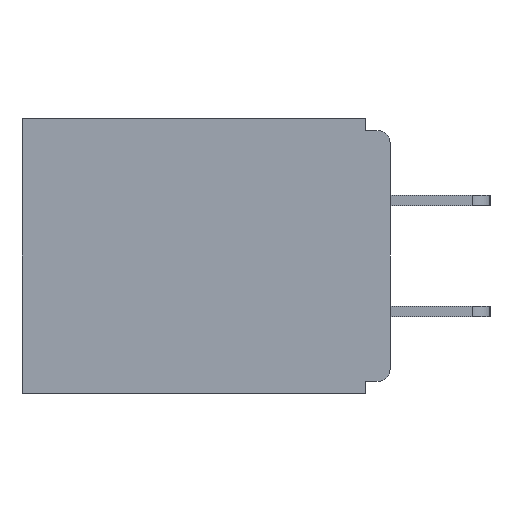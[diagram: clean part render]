
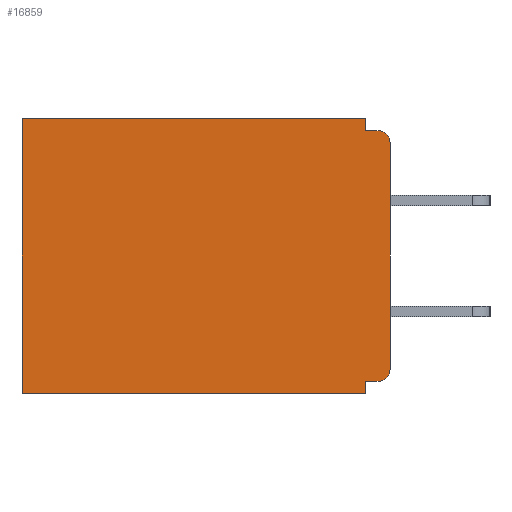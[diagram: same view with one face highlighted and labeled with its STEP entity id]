
A CAD part, left-side view. The second image highlights one B-rep face of the part: STEP entity #16859.
In plain terms, the highlighted planar face has unit normal (-1, 0, 0).
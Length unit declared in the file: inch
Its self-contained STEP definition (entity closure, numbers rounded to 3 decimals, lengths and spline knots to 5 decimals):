
#221 = EDGE_CURVE ( 'NONE', #4539, #14338, #4258, .T. ) ;
#239 = DIRECTION ( 'NONE',  ( 0., 0., -1. ) ) ;
#293 = DIRECTION ( 'NONE',  ( -1., 0., 0. ) ) ;
#510 = ORIENTED_EDGE ( 'NONE', *, *, #3918, .T. ) ;
#645 = VECTOR ( 'NONE', #3344, 39.37008 ) ;
#676 = PLANE ( 'NONE',  #13515 ) ;
#951 = ORIENTED_EDGE ( 'NONE', *, *, #10833, .F. ) ;
#1145 = ORIENTED_EDGE ( 'NONE', *, *, #6281, .T. ) ;
#1488 = CARTESIAN_POINT ( 'NONE',  ( 0.298, 0.015, -0.313 ) ) ;
#2390 = VERTEX_POINT ( 'NONE', #12334 ) ;
#2762 = EDGE_LOOP ( 'NONE', ( #510, #6011, #5870, #3075, #7403, #951, #15896, #7217, #1145, #3067 ) ) ;
#2791 = CIRCLE ( 'NONE', #11341, 0.015 ) ;
#2905 = EDGE_CURVE ( 'NONE', #3088, #14174, #4591, .T. ) ;
#3053 = AXIS2_PLACEMENT_3D ( 'NONE', #12377, #16172, #12255 ) ;
#3055 = EDGE_CURVE ( 'NONE', #2390, #16851, #3716, .T. ) ;
#3067 = ORIENTED_EDGE ( 'NONE', *, *, #2905, .F. ) ;
#3075 = ORIENTED_EDGE ( 'NONE', *, *, #9338, .T. ) ;
#3088 = VERTEX_POINT ( 'NONE', #14588 ) ;
#3344 = DIRECTION ( 'NONE',  ( 0., 1., 0. ) ) ;
#3475 = EDGE_CURVE ( 'NONE', #16851, #15355, #7860, .T. ) ;
#3716 = LINE ( 'NONE', #17116, #13738 ) ;
#3918 = EDGE_CURVE ( 'NONE', #3088, #15355, #13923, .T. ) ;
#3971 = LINE ( 'NONE', #9865, #645 ) ;
#3990 = LINE ( 'NONE', #4992, #15220 ) ;
#4104 = CARTESIAN_POINT ( 'NONE',  ( 0.298, 0.015, -0.328 ) ) ;
#4258 = LINE ( 'NONE', #12077, #7594 ) ;
#4539 = VERTEX_POINT ( 'NONE', #4104 ) ;
#4559 = LINE ( 'NONE', #13170, #6616 ) ;
#4591 = LINE ( 'NONE', #14930, #13950 ) ;
#4704 = DIRECTION ( 'NONE',  ( 0., 0., -1. ) ) ;
#4992 = CARTESIAN_POINT ( 'NONE',  ( 0.298, 0.031, -0.343 ) ) ;
#5870 = ORIENTED_EDGE ( 'NONE', *, *, #3055, .F. ) ;
#5991 = CARTESIAN_POINT ( 'NONE',  ( 0.298, 0., 0. ) ) ;
#6011 = ORIENTED_EDGE ( 'NONE', *, *, #3475, .F. ) ;
#6237 = DIRECTION ( 'NONE',  ( 0., 0., -1. ) ) ;
#6281 = EDGE_CURVE ( 'NONE', #4539, #14174, #2791, .T. ) ;
#6289 = VERTEX_POINT ( 'NONE', #13451 ) ;
#6616 = VECTOR ( 'NONE', #7856, 39.37008 ) ;
#6645 = CARTESIAN_POINT ( 'NONE',  ( 0.298, 0.46, -0.343 ) ) ;
#7136 = LINE ( 'NONE', #9548, #13598 ) ;
#7217 = ORIENTED_EDGE ( 'NONE', *, *, #221, .F. ) ;
#7403 = ORIENTED_EDGE ( 'NONE', *, *, #17065, .T. ) ;
#7594 = VECTOR ( 'NONE', #16400, 39.37008 ) ;
#7681 = CARTESIAN_POINT ( 'NONE',  ( 0.298, 0.015, -0.015 ) ) ;
#7856 = DIRECTION ( 'NONE',  ( 0., 0., -1. ) ) ;
#7860 = LINE ( 'NONE', #15106, #12038 ) ;
#8311 = DIRECTION ( 'NONE',  ( 0., 0., -1. ) ) ;
#8358 = DIRECTION ( 'NONE',  ( 0., -1., 0. ) ) ;
#8578 = CARTESIAN_POINT ( 'NONE',  ( 0.298, 0.031, -0.015 ) ) ;
#9195 = VERTEX_POINT ( 'NONE', #10672 ) ;
#9338 = EDGE_CURVE ( 'NONE', #2390, #9195, #7136, .T. ) ;
#9548 = CARTESIAN_POINT ( 'NONE',  ( 0.298, 0., 0. ) ) ;
#9865 = CARTESIAN_POINT ( 'NONE',  ( 0.298, 0., -0.343 ) ) ;
#10512 = EDGE_CURVE ( 'NONE', #14338, #6289, #3990, .T. ) ;
#10605 = VERTEX_POINT ( 'NONE', #6645 ) ;
#10672 = CARTESIAN_POINT ( 'NONE',  ( 0.298, 0.46, 0. ) ) ;
#10833 = EDGE_CURVE ( 'NONE', #6289, #10605, #3971, .T. ) ;
#11341 = AXIS2_PLACEMENT_3D ( 'NONE', #1488, #293, #239 ) ;
#12038 = VECTOR ( 'NONE', #8358, 39.37008 ) ;
#12077 = CARTESIAN_POINT ( 'NONE',  ( 0.298, 0., -0.328 ) ) ;
#12170 = CARTESIAN_POINT ( 'NONE',  ( 0.298, 0.031, -0.328 ) ) ;
#12255 = DIRECTION ( 'NONE',  ( 0., 0., -1. ) ) ;
#12334 = CARTESIAN_POINT ( 'NONE',  ( 0.298, 0.031, 0. ) ) ;
#12377 = CARTESIAN_POINT ( 'NONE',  ( 0.298, 0.015, -0.03 ) ) ;
#12614 = DIRECTION ( 'NONE',  ( 1., 0., 0. ) ) ;
#13156 = CARTESIAN_POINT ( 'NONE',  ( 0.298, 0., -0.313 ) ) ;
#13170 = CARTESIAN_POINT ( 'NONE',  ( 0.298, 0.46, 0. ) ) ;
#13451 = CARTESIAN_POINT ( 'NONE',  ( 0.298, 0.031, -0.343 ) ) ;
#13515 = AXIS2_PLACEMENT_3D ( 'NONE', #5991, #12614, #4704 ) ;
#13598 = VECTOR ( 'NONE', #13766, 39.37008 ) ;
#13738 = VECTOR ( 'NONE', #6237, 39.37008 ) ;
#13766 = DIRECTION ( 'NONE',  ( 0., 1., 0. ) ) ;
#13923 = CIRCLE ( 'NONE', #3053, 0.015 ) ;
#13950 = VECTOR ( 'NONE', #8311, 39.37008 ) ;
#14174 = VERTEX_POINT ( 'NONE', #13156 ) ;
#14338 = VERTEX_POINT ( 'NONE', #12170 ) ;
#14588 = CARTESIAN_POINT ( 'NONE',  ( 0.298, 0., -0.03 ) ) ;
#14930 = CARTESIAN_POINT ( 'NONE',  ( 0.298, 0., 0. ) ) ;
#15106 = CARTESIAN_POINT ( 'NONE',  ( 0.298, 0., -0.015 ) ) ;
#15220 = VECTOR ( 'NONE', #17031, 39.37008 ) ;
#15355 = VERTEX_POINT ( 'NONE', #7681 ) ;
#15896 = ORIENTED_EDGE ( 'NONE', *, *, #10512, .F. ) ;
#16172 = DIRECTION ( 'NONE',  ( -1., 0., 0. ) ) ;
#16400 = DIRECTION ( 'NONE',  ( 0., 1., 0. ) ) ;
#16812 = FACE_OUTER_BOUND ( 'NONE', #2762, .T. ) ;
#16851 = VERTEX_POINT ( 'NONE', #8578 ) ;
#16859 = ADVANCED_FACE ( 'NONE', ( #16812 ), #676, .F. ) ;
#17031 = DIRECTION ( 'NONE',  ( 0., 0., -1. ) ) ;
#17065 = EDGE_CURVE ( 'NONE', #9195, #10605, #4559, .T. ) ;
#17116 = CARTESIAN_POINT ( 'NONE',  ( 0.298, 0.031, -0.343 ) ) ;
